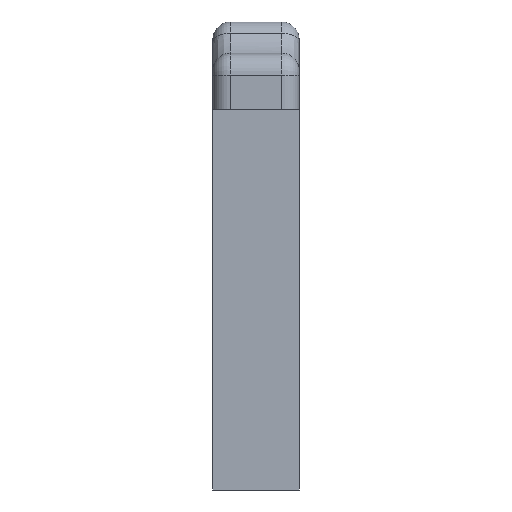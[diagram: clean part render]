
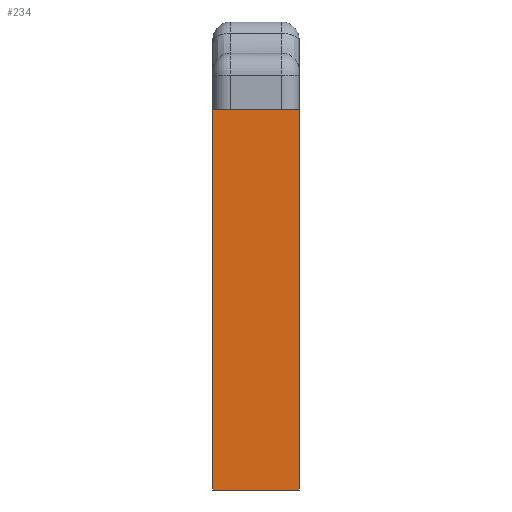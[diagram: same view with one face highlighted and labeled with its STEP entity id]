
A CAD part, front view. The second image highlights one B-rep face of the part: STEP entity #234.
In plain terms, the highlighted planar face has unit normal (0, -1, 0).
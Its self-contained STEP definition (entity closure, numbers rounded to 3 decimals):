
#34 = EDGE_CURVE ( 'NONE', #1578, #1037, #838, .T. ) ;
#234 = ADVANCED_FACE ( 'NONE', ( #746 ), #554, .F. ) ;
#261 = CARTESIAN_POINT ( 'NONE',  ( 9.898, -2.5, 5. ) ) ;
#286 = CARTESIAN_POINT ( 'NONE',  ( 0., -2.5, 15. ) ) ;
#287 = DIRECTION ( 'NONE',  ( 0., 1., 0. ) ) ;
#311 = DIRECTION ( 'NONE',  ( 0., 0., 1. ) ) ;
#379 = VECTOR ( 'NONE', #1033, 1000. ) ;
#421 = EDGE_LOOP ( 'NONE', ( #1050, #1235, #1280, #1359 ) ) ;
#422 = LINE ( 'NONE', #899, #379 ) ;
#456 = VECTOR ( 'NONE', #983, 1000. ) ;
#458 = LINE ( 'NONE', #261, #456 ) ;
#504 = CARTESIAN_POINT ( 'NONE',  ( 9.898, -2.5, -38.75 ) ) ;
#526 = VECTOR ( 'NONE', #837, 1000. ) ;
#548 = LINE ( 'NONE', #1355, #526 ) ;
#554 = PLANE ( 'NONE',  #1061 ) ;
#746 = FACE_OUTER_BOUND ( 'NONE', #421, .T. ) ;
#784 = EDGE_CURVE ( 'NONE', #1644, #1316, #548, .T. ) ;
#835 = VECTOR ( 'NONE', #1205, 1000. ) ;
#837 = DIRECTION ( 'NONE',  ( 0., 0., -1. ) ) ;
#838 = LINE ( 'NONE', #286, #835 ) ;
#899 = CARTESIAN_POINT ( 'NONE',  ( 9.898, -2.5, -38.75 ) ) ;
#983 = DIRECTION ( 'NONE',  ( 1., 0., 0. ) ) ;
#995 = EDGE_CURVE ( 'NONE', #1578, #1644, #458, .T. ) ;
#1033 = DIRECTION ( 'NONE',  ( -1., 0., 0. ) ) ;
#1037 = VERTEX_POINT ( 'NONE', #1629 ) ;
#1050 = ORIENTED_EDGE ( 'NONE', *, *, #995, .F. ) ;
#1061 = AXIS2_PLACEMENT_3D ( 'NONE', #1077, #287, #311 ) ;
#1077 = CARTESIAN_POINT ( 'NONE',  ( 9.898, -2.5, 15. ) ) ;
#1106 = CARTESIAN_POINT ( 'NONE',  ( 0., -2.5, 5. ) ) ;
#1131 = CARTESIAN_POINT ( 'NONE',  ( 9.898, -2.5, 5. ) ) ;
#1205 = DIRECTION ( 'NONE',  ( 0., 0., -1. ) ) ;
#1212 = EDGE_CURVE ( 'NONE', #1316, #1037, #422, .T. ) ;
#1235 = ORIENTED_EDGE ( 'NONE', *, *, #34, .T. ) ;
#1280 = ORIENTED_EDGE ( 'NONE', *, *, #1212, .F. ) ;
#1316 = VERTEX_POINT ( 'NONE', #504 ) ;
#1355 = CARTESIAN_POINT ( 'NONE',  ( 9.898, -2.5, 15. ) ) ;
#1359 = ORIENTED_EDGE ( 'NONE', *, *, #784, .F. ) ;
#1578 = VERTEX_POINT ( 'NONE', #1106 ) ;
#1629 = CARTESIAN_POINT ( 'NONE',  ( 0., -2.5, -38.75 ) ) ;
#1644 = VERTEX_POINT ( 'NONE', #1131 ) ;
